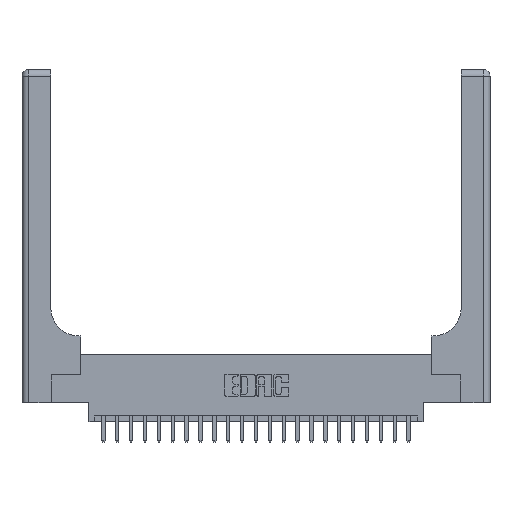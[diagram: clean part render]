
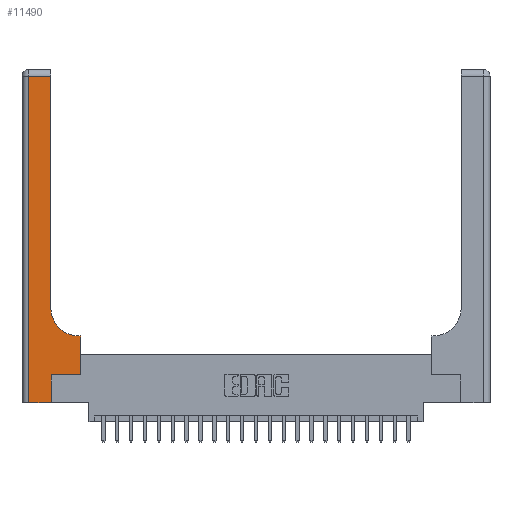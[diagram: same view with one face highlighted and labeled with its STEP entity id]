
A CAD part, top view. The second image highlights one B-rep face of the part: STEP entity #11490.
In plain terms, the highlighted planar face has unit normal (0, 0, 1).
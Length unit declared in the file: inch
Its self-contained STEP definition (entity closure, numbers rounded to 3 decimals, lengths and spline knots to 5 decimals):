
#209 = DIRECTION ( 'NONE',  ( -1., 0., 0. ) ) ;
#1327 = ORIENTED_EDGE ( 'NONE', *, *, #12608, .T. ) ;
#2064 = ORIENTED_EDGE ( 'NONE', *, *, #12260, .T. ) ;
#2197 = VERTEX_POINT ( 'NONE', #11722 ) ;
#2223 = EDGE_CURVE ( 'NONE', #2197, #21793, #12340, .T. ) ;
#2778 = LINE ( 'NONE', #21610, #7227 ) ;
#3281 = LINE ( 'NONE', #20378, #21524 ) ;
#3528 = EDGE_LOOP ( 'NONE', ( #17896, #17541, #1327, #2064, #10931, #7283, #18362, #9603, #11260 ) ) ;
#3862 = PLANE ( 'NONE',  #13523 ) ;
#4319 = VERTEX_POINT ( 'NONE', #15114 ) ;
#4747 = CARTESIAN_POINT ( 'NONE',  ( 0.06, 3., 0.37 ) ) ;
#5800 = CARTESIAN_POINT ( 'NONE',  ( 0., 3., 0.37 ) ) ;
#6219 = VERTEX_POINT ( 'NONE', #16515 ) ;
#6504 = VECTOR ( 'NONE', #19610, 39.37008 ) ;
#6881 = VECTOR ( 'NONE', #10623, 39.37008 ) ;
#6919 = VECTOR ( 'NONE', #8448, 39.37008 ) ;
#7227 = VECTOR ( 'NONE', #209, 39.37008 ) ;
#7283 = ORIENTED_EDGE ( 'NONE', *, *, #2223, .T. ) ;
#7373 = AXIS2_PLACEMENT_3D ( 'NONE', #10524, #22389, #12332 ) ;
#7670 = DIRECTION ( 'NONE',  ( 0., 0., -1. ) ) ;
#8332 = EDGE_CURVE ( 'NONE', #19217, #18620, #11169, .T. ) ;
#8448 = DIRECTION ( 'NONE',  ( 0., -1., 0. ) ) ;
#8958 = CARTESIAN_POINT ( 'NONE',  ( 0., 0., 0.37 ) ) ;
#8970 = DIRECTION ( 'NONE',  ( 0., 1., 0. ) ) ;
#9055 = CARTESIAN_POINT ( 'NONE',  ( 0.26, 0.85, 0.37 ) ) ;
#9603 = ORIENTED_EDGE ( 'NONE', *, *, #13059, .T. ) ;
#10025 = CARTESIAN_POINT ( 'NONE',  ( 0.06, 0., 0.37 ) ) ;
#10524 = CARTESIAN_POINT ( 'NONE',  ( 0.51, 0.85, 0.37 ) ) ;
#10623 = DIRECTION ( 'NONE',  ( 1., 0., 0. ) ) ;
#10732 = CARTESIAN_POINT ( 'NONE',  ( 0.265, 0.25, 0.37 ) ) ;
#10931 = ORIENTED_EDGE ( 'NONE', *, *, #15467, .T. ) ;
#11169 = CIRCLE ( 'NONE', #7373, 0.25 ) ;
#11260 = ORIENTED_EDGE ( 'NONE', *, *, #8332, .T. ) ;
#11490 = ADVANCED_FACE ( 'NONE', ( #14080 ), #3862, .F. ) ;
#11722 = CARTESIAN_POINT ( 'NONE',  ( 0.265, 0.25, 0.37 ) ) ;
#12260 = EDGE_CURVE ( 'NONE', #18976, #22391, #22110, .T. ) ;
#12332 = DIRECTION ( 'NONE',  ( 1., 0., 0. ) ) ;
#12340 = LINE ( 'NONE', #10732, #6881 ) ;
#12608 = EDGE_CURVE ( 'NONE', #19719, #18976, #20317, .T. ) ;
#12618 = DIRECTION ( 'NONE',  ( 1., 0., 0. ) ) ;
#13043 = LINE ( 'NONE', #13874, #17502 ) ;
#13059 = EDGE_CURVE ( 'NONE', #4319, #19217, #2778, .T. ) ;
#13230 = VECTOR ( 'NONE', #12618, 39.37008 ) ;
#13523 = AXIS2_PLACEMENT_3D ( 'NONE', #5800, #7670, #19884 ) ;
#13738 = DIRECTION ( 'NONE',  ( 0., 1., 0. ) ) ;
#13874 = CARTESIAN_POINT ( 'NONE',  ( 0.26, 3., 0.37 ) ) ;
#13936 = EDGE_CURVE ( 'NONE', #21793, #4319, #3281, .T. ) ;
#14080 = FACE_OUTER_BOUND ( 'NONE', #3528, .T. ) ;
#14738 = LINE ( 'NONE', #22660, #18666 ) ;
#15114 = CARTESIAN_POINT ( 'NONE',  ( 0.528, 0.6, 0.37 ) ) ;
#15467 = EDGE_CURVE ( 'NONE', #22391, #2197, #14738, .T. ) ;
#16515 = CARTESIAN_POINT ( 'NONE',  ( 0.26, 2.94, 0.37 ) ) ;
#17109 = CARTESIAN_POINT ( 'NONE',  ( 0.528, 0.25, 0.37 ) ) ;
#17502 = VECTOR ( 'NONE', #20516, 39.37008 ) ;
#17541 = ORIENTED_EDGE ( 'NONE', *, *, #20366, .T. ) ;
#17686 = CARTESIAN_POINT ( 'NONE',  ( 0.06, 2.94, 0.37 ) ) ;
#17882 = CARTESIAN_POINT ( 'NONE',  ( 0., 2.94, 0.37 ) ) ;
#17896 = ORIENTED_EDGE ( 'NONE', *, *, #21164, .T. ) ;
#18362 = ORIENTED_EDGE ( 'NONE', *, *, #13936, .T. ) ;
#18620 = VERTEX_POINT ( 'NONE', #9055 ) ;
#18666 = VECTOR ( 'NONE', #8970, 39.37008 ) ;
#18976 = VERTEX_POINT ( 'NONE', #10025 ) ;
#19027 = CARTESIAN_POINT ( 'NONE',  ( 0.265, 0., 0.37 ) ) ;
#19217 = VERTEX_POINT ( 'NONE', #22853 ) ;
#19610 = DIRECTION ( 'NONE',  ( -1., 0., 0. ) ) ;
#19719 = VERTEX_POINT ( 'NONE', #17686 ) ;
#19884 = DIRECTION ( 'NONE',  ( -1., 0., 0. ) ) ;
#20317 = LINE ( 'NONE', #4747, #6919 ) ;
#20366 = EDGE_CURVE ( 'NONE', #6219, #19719, #20440, .T. ) ;
#20378 = CARTESIAN_POINT ( 'NONE',  ( 0.528, 0.25, 0.37 ) ) ;
#20440 = LINE ( 'NONE', #17882, #6504 ) ;
#20516 = DIRECTION ( 'NONE',  ( 0., 1., 0. ) ) ;
#21164 = EDGE_CURVE ( 'NONE', #18620, #6219, #13043, .T. ) ;
#21524 = VECTOR ( 'NONE', #13738, 39.37008 ) ;
#21610 = CARTESIAN_POINT ( 'NONE',  ( 0.26, 0.6, 0.37 ) ) ;
#21793 = VERTEX_POINT ( 'NONE', #17109 ) ;
#22110 = LINE ( 'NONE', #8958, #13230 ) ;
#22389 = DIRECTION ( 'NONE',  ( 0., 0., -1. ) ) ;
#22391 = VERTEX_POINT ( 'NONE', #19027 ) ;
#22660 = CARTESIAN_POINT ( 'NONE',  ( 0.265, 0., 0.37 ) ) ;
#22853 = CARTESIAN_POINT ( 'NONE',  ( 0.51, 0.6, 0.37 ) ) ;
